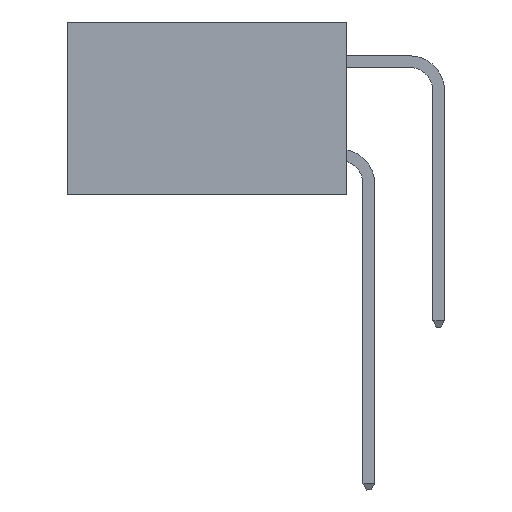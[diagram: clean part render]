
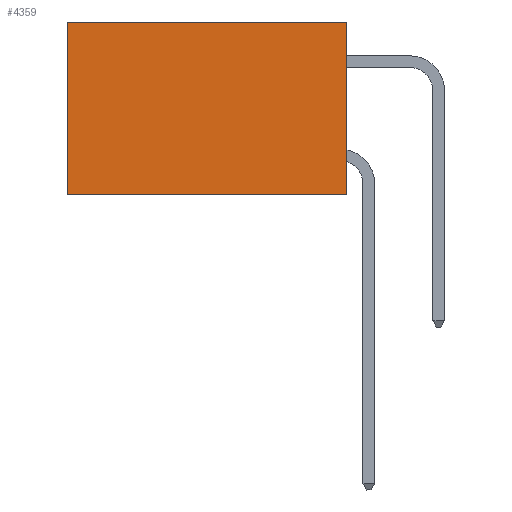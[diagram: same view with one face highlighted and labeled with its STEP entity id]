
A CAD part, left-side view. The second image highlights one B-rep face of the part: STEP entity #4359.
In plain terms, the highlighted planar face has unit normal (-1, 0, 0).
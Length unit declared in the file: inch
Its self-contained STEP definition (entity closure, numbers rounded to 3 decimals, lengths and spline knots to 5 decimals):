
#465 = FACE_OUTER_BOUND ( 'NONE', #9971, .T. ) ;
#665 = EDGE_CURVE ( 'NONE', #7947, #3403, #10004, .T. ) ;
#978 = VECTOR ( 'NONE', #4908, 39.37008 ) ;
#1306 = LINE ( 'NONE', #7319, #978 ) ;
#2334 = LINE ( 'NONE', #9268, #6639 ) ;
#2400 = VERTEX_POINT ( 'NONE', #9540 ) ;
#2835 = VERTEX_POINT ( 'NONE', #5320 ) ;
#2899 = VECTOR ( 'NONE', #3701, 39.37008 ) ;
#3017 = EDGE_CURVE ( 'NONE', #7947, #2400, #7633, .T. ) ;
#3289 = CARTESIAN_POINT ( 'NONE',  ( 0.2875, 0.6, 0. ) ) ;
#3403 = VERTEX_POINT ( 'NONE', #3289 ) ;
#3601 = DIRECTION ( 'NONE',  ( 0., 1., 0. ) ) ;
#3687 = CARTESIAN_POINT ( 'NONE',  ( 0.2875, 0., 0. ) ) ;
#3701 = DIRECTION ( 'NONE',  ( 0., 0., -1. ) ) ;
#3792 = AXIS2_PLACEMENT_3D ( 'NONE', #6109, #6423, #7045 ) ;
#4155 = EDGE_CURVE ( 'NONE', #3403, #2835, #1306, .T. ) ;
#4359 = ADVANCED_FACE ( 'NONE', ( #465 ), #6197, .F. ) ;
#4908 = DIRECTION ( 'NONE',  ( 0., 0., -1. ) ) ;
#5320 = CARTESIAN_POINT ( 'NONE',  ( 0.2875, 0.6, -0.37 ) ) ;
#5424 = ORIENTED_EDGE ( 'NONE', *, *, #8109, .F. ) ;
#5998 = DIRECTION ( 'NONE',  ( 0., 1., 0. ) ) ;
#6109 = CARTESIAN_POINT ( 'NONE',  ( 0.2875, 0., 0. ) ) ;
#6197 = PLANE ( 'NONE',  #3792 ) ;
#6243 = ORIENTED_EDGE ( 'NONE', *, *, #4155, .T. ) ;
#6423 = DIRECTION ( 'NONE',  ( 1., 0., 0. ) ) ;
#6639 = VECTOR ( 'NONE', #3601, 39.37008 ) ;
#6701 = ORIENTED_EDGE ( 'NONE', *, *, #3017, .F. ) ;
#6722 = CARTESIAN_POINT ( 'NONE',  ( 0.2875, 0., 0. ) ) ;
#7045 = DIRECTION ( 'NONE',  ( 0., 0., -1. ) ) ;
#7319 = CARTESIAN_POINT ( 'NONE',  ( 0.2875, 0.6, 0. ) ) ;
#7633 = LINE ( 'NONE', #3687, #2899 ) ;
#7802 = VECTOR ( 'NONE', #5998, 39.37008 ) ;
#7947 = VERTEX_POINT ( 'NONE', #10509 ) ;
#8109 = EDGE_CURVE ( 'NONE', #2400, #2835, #2334, .T. ) ;
#9268 = CARTESIAN_POINT ( 'NONE',  ( 0.2875, 0., -0.37 ) ) ;
#9540 = CARTESIAN_POINT ( 'NONE',  ( 0.2875, 0., -0.37 ) ) ;
#9866 = ORIENTED_EDGE ( 'NONE', *, *, #665, .T. ) ;
#9971 = EDGE_LOOP ( 'NONE', ( #6243, #5424, #6701, #9866 ) ) ;
#10004 = LINE ( 'NONE', #6722, #7802 ) ;
#10509 = CARTESIAN_POINT ( 'NONE',  ( 0.2875, 0., 0. ) ) ;
